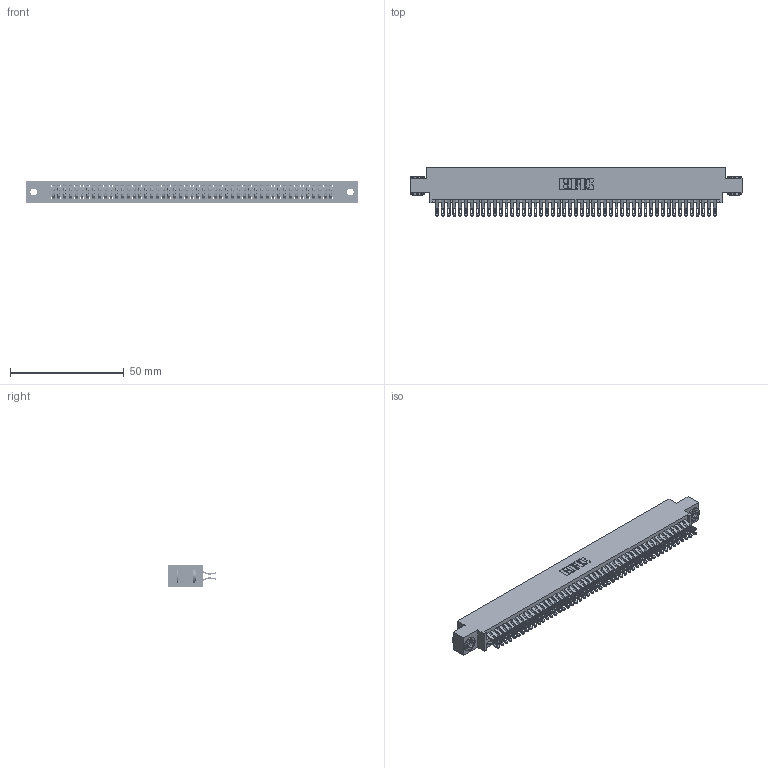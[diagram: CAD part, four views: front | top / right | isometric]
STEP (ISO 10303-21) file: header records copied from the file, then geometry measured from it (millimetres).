
FILE_DESCRIPTION (( 'STEP AP203' ), '1' );
FILE_NAME ('395-098-555-803.STEP', '2018-11-29T21:46:09', ( '' ), ( '' ), 'SwSTEP 2.0', 'SolidWorks 2016', '' );
FILE_SCHEMA (( 'CONFIG_CONTROL_DESIGN' ));
Length unit declared in the file: inch
Products named in the file (4): 345-250-002_345-250-002-102; 345 Part_0.170 Offset - 0.156 Dia-TH; 345-292-001_555 Tail; 395-098-555-803
Assembly tree (101 placements, depth 2):
  395-098-555-803
    345 Part_0.170 Offset - 0.156 Dia-TH
    345-292-001_555 Tail  x98
    345-250-002_345-250-002-102  x2
Bounding box: 145.67 x 21.13 x 9.4 mm (x, y, z)
Volume: 14405.7 mm3; surface area: 22766.6 mm2
Topology: 101 solids, 101 shells, 5656 faces, 17775 edges, 11846 vertices
Faces by surface type: plane 3132, cylinder 2516, cone 8
Entity records: 38612 total; most frequent: CARTESIAN_POINT 6477, ORIENTED_EDGE 6374, DIRECTION 5701, EDGE_CURVE 3187, LINE 2815, VECTOR 2815, VERTEX_POINT 2122, AXIS2_PLACEMENT_3D 1443
